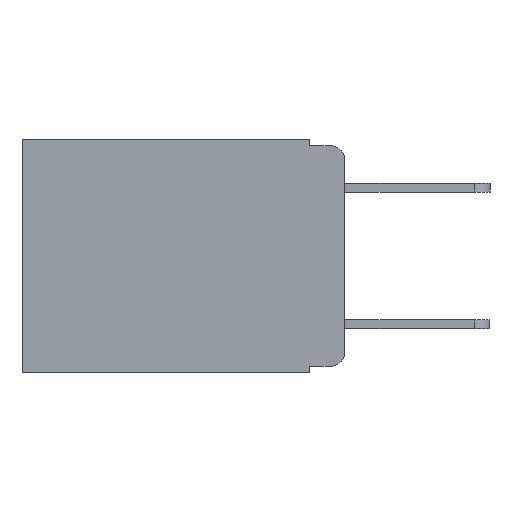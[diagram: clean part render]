
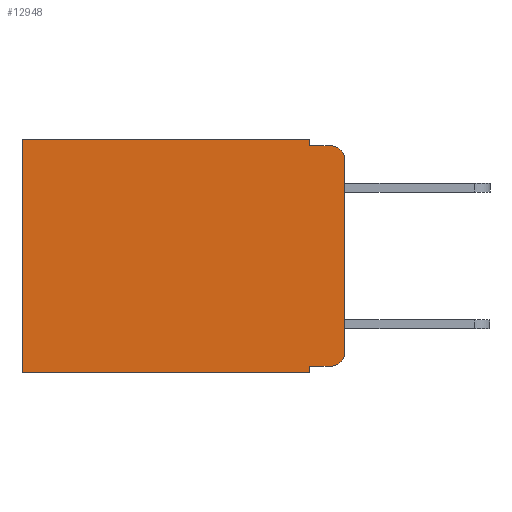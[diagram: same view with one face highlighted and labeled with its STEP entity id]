
A CAD part, left-side view. The second image highlights one B-rep face of the part: STEP entity #12948.
In plain terms, the highlighted planar face has unit normal (-1, 0, 0).
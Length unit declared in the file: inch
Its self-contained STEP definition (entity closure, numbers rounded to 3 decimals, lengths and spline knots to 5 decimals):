
#310 = CARTESIAN_POINT ( 'NONE',  ( 0.298, 0.473, 0. ) ) ;
#312 = CARTESIAN_POINT ( 'NONE',  ( 0.298, 0., -0.343 ) ) ;
#365 = CIRCLE ( 'NONE', #6317, 0.02 ) ;
#1462 = EDGE_CURVE ( 'NONE', #12920, #10793, #19463, .T. ) ;
#1596 = VECTOR ( 'NONE', #7568, 39.37008 ) ;
#1838 = DIRECTION ( 'NONE',  ( -1., 0., 0. ) ) ;
#1976 = ORIENTED_EDGE ( 'NONE', *, *, #19714, .T. ) ;
#2275 = DIRECTION ( 'NONE',  ( 0., 0., -1. ) ) ;
#2411 = CARTESIAN_POINT ( 'NONE',  ( 0.298, 0.473, -0.343 ) ) ;
#2415 = EDGE_CURVE ( 'NONE', #10793, #21818, #365, .T. ) ;
#2887 = VECTOR ( 'NONE', #2275, 39.37008 ) ;
#3142 = ORIENTED_EDGE ( 'NONE', *, *, #10066, .F. ) ;
#3546 = VERTEX_POINT ( 'NONE', #4492 ) ;
#3628 = CARTESIAN_POINT ( 'NONE',  ( 0.298, 0.02, -0.01 ) ) ;
#4172 = VECTOR ( 'NONE', #16202, 39.37008 ) ;
#4492 = CARTESIAN_POINT ( 'NONE',  ( 0.298, 0.051, -0.343 ) ) ;
#4494 = CARTESIAN_POINT ( 'NONE',  ( 0.298, 0., -0.313 ) ) ;
#4666 = CIRCLE ( 'NONE', #20470, 0.02 ) ;
#4788 = LINE ( 'NONE', #7168, #4172 ) ;
#4815 = DIRECTION ( 'NONE',  ( 1., 0., 0. ) ) ;
#5405 = EDGE_CURVE ( 'NONE', #12920, #3546, #11111, .T. ) ;
#5639 = VERTEX_POINT ( 'NONE', #17430 ) ;
#6317 = AXIS2_PLACEMENT_3D ( 'NONE', #9953, #9906, #22737 ) ;
#6604 = AXIS2_PLACEMENT_3D ( 'NONE', #20952, #4815, #17582 ) ;
#7168 = CARTESIAN_POINT ( 'NONE',  ( 0.298, 0., 0. ) ) ;
#7568 = DIRECTION ( 'NONE',  ( 0., 0., -1. ) ) ;
#7856 = VERTEX_POINT ( 'NONE', #2411 ) ;
#8914 = VERTEX_POINT ( 'NONE', #9451 ) ;
#9052 = ORIENTED_EDGE ( 'NONE', *, *, #20638, .T. ) ;
#9357 = ORIENTED_EDGE ( 'NONE', *, *, #5405, .F. ) ;
#9400 = CARTESIAN_POINT ( 'NONE',  ( 0.298, 0., 0. ) ) ;
#9451 = CARTESIAN_POINT ( 'NONE',  ( 0.298, 0., -0.03 ) ) ;
#9571 = DIRECTION ( 'NONE',  ( 0., -1., 0. ) ) ;
#9762 = LINE ( 'NONE', #10446, #14034 ) ;
#9906 = DIRECTION ( 'NONE',  ( -1., 0., 0. ) ) ;
#9953 = CARTESIAN_POINT ( 'NONE',  ( 0.298, 0.02, -0.313 ) ) ;
#9979 = VECTOR ( 'NONE', #9571, 39.37008 ) ;
#10066 = EDGE_CURVE ( 'NONE', #19112, #21551, #14242, .T. ) ;
#10116 = FACE_OUTER_BOUND ( 'NONE', #12737, .T. ) ;
#10256 = CARTESIAN_POINT ( 'NONE',  ( 0.298, 0.051, -0.333 ) ) ;
#10446 = CARTESIAN_POINT ( 'NONE',  ( 0.298, 0.051, 0. ) ) ;
#10793 = VERTEX_POINT ( 'NONE', #16596 ) ;
#10804 = EDGE_CURVE ( 'NONE', #8914, #21818, #11633, .T. ) ;
#11111 = LINE ( 'NONE', #12875, #20004 ) ;
#11312 = VECTOR ( 'NONE', #17107, 39.37008 ) ;
#11505 = EDGE_CURVE ( 'NONE', #3546, #7856, #16119, .T. ) ;
#11616 = CARTESIAN_POINT ( 'NONE',  ( 0.298, 0.051, -0.01 ) ) ;
#11633 = LINE ( 'NONE', #9400, #1596 ) ;
#11860 = ORIENTED_EDGE ( 'NONE', *, *, #11505, .F. ) ;
#12737 = EDGE_LOOP ( 'NONE', ( #17546, #18821, #3142, #22344, #1976, #9052, #11860, #9357, #21632, #22220 ) ) ;
#12820 = LINE ( 'NONE', #310, #2887 ) ;
#12875 = CARTESIAN_POINT ( 'NONE',  ( 0.298, 0.051, 0. ) ) ;
#12885 = CARTESIAN_POINT ( 'NONE',  ( 0.298, 0.473, 0. ) ) ;
#12920 = VERTEX_POINT ( 'NONE', #10256 ) ;
#12948 = ADVANCED_FACE ( 'NONE', ( #10116 ), #15782, .F. ) ;
#13104 = CARTESIAN_POINT ( 'NONE',  ( 0.298, 0.02, -0.03 ) ) ;
#14034 = VECTOR ( 'NONE', #22791, 39.37008 ) ;
#14242 = LINE ( 'NONE', #19815, #22945 ) ;
#14902 = DIRECTION ( 'NONE',  ( 0., 0., -1. ) ) ;
#15234 = EDGE_CURVE ( 'NONE', #5639, #19112, #9762, .T. ) ;
#15745 = CARTESIAN_POINT ( 'NONE',  ( 0.298, 0.051, -0.333 ) ) ;
#15782 = PLANE ( 'NONE',  #6604 ) ;
#16075 = VERTEX_POINT ( 'NONE', #12885 ) ;
#16119 = LINE ( 'NONE', #312, #11312 ) ;
#16202 = DIRECTION ( 'NONE',  ( 0., 1., 0. ) ) ;
#16562 = EDGE_CURVE ( 'NONE', #8914, #21551, #4666, .T. ) ;
#16596 = CARTESIAN_POINT ( 'NONE',  ( 0.298, 0.02, -0.333 ) ) ;
#17107 = DIRECTION ( 'NONE',  ( 0., 1., 0. ) ) ;
#17430 = CARTESIAN_POINT ( 'NONE',  ( 0.298, 0.051, 0. ) ) ;
#17546 = ORIENTED_EDGE ( 'NONE', *, *, #10804, .F. ) ;
#17582 = DIRECTION ( 'NONE',  ( 0., 0., -1. ) ) ;
#18821 = ORIENTED_EDGE ( 'NONE', *, *, #16562, .T. ) ;
#19112 = VERTEX_POINT ( 'NONE', #11616 ) ;
#19463 = LINE ( 'NONE', #15745, #9979 ) ;
#19714 = EDGE_CURVE ( 'NONE', #5639, #16075, #4788, .T. ) ;
#19815 = CARTESIAN_POINT ( 'NONE',  ( 0.298, 0.051, -0.01 ) ) ;
#20004 = VECTOR ( 'NONE', #22922, 39.37008 ) ;
#20470 = AXIS2_PLACEMENT_3D ( 'NONE', #13104, #1838, #14902 ) ;
#20638 = EDGE_CURVE ( 'NONE', #16075, #7856, #12820, .T. ) ;
#20952 = CARTESIAN_POINT ( 'NONE',  ( 0.298, 0., 0. ) ) ;
#21551 = VERTEX_POINT ( 'NONE', #3628 ) ;
#21567 = DIRECTION ( 'NONE',  ( 0., -1., 0. ) ) ;
#21632 = ORIENTED_EDGE ( 'NONE', *, *, #1462, .T. ) ;
#21818 = VERTEX_POINT ( 'NONE', #4494 ) ;
#22220 = ORIENTED_EDGE ( 'NONE', *, *, #2415, .T. ) ;
#22344 = ORIENTED_EDGE ( 'NONE', *, *, #15234, .F. ) ;
#22737 = DIRECTION ( 'NONE',  ( 0., 0., -1. ) ) ;
#22791 = DIRECTION ( 'NONE',  ( 0., 0., -1. ) ) ;
#22922 = DIRECTION ( 'NONE',  ( 0., 0., -1. ) ) ;
#22945 = VECTOR ( 'NONE', #21567, 39.37008 ) ;
